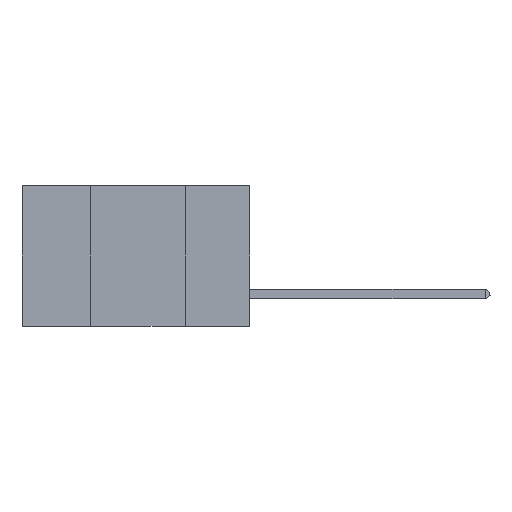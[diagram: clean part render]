
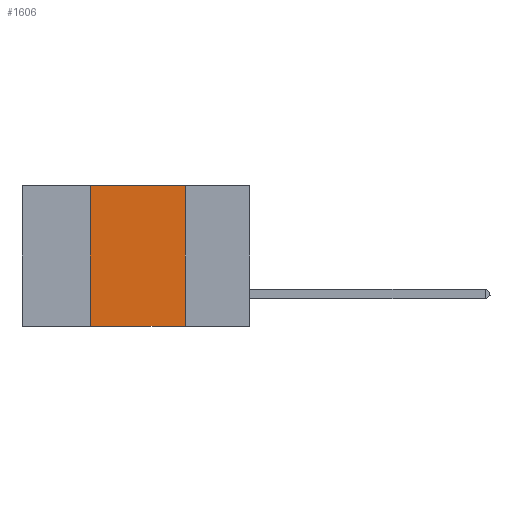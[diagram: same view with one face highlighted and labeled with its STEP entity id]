
A CAD part, left-side view. The second image highlights one B-rep face of the part: STEP entity #1606.
In plain terms, the highlighted planar face has unit normal (-1, 0, 0).
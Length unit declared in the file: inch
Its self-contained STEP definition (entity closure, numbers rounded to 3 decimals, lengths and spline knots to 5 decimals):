
#1122 = DIRECTION ( 'NONE',  ( 0., 0., 1. ) ) ;
#1606 = ADVANCED_FACE ( 'NONE', ( #5337 ), #13560, .F. ) ;
#1828 = VECTOR ( 'NONE', #7093, 39.37008 ) ;
#2267 = VECTOR ( 'NONE', #9466, 39.37008 ) ;
#2295 = DIRECTION ( 'NONE',  ( 0., 0., -1. ) ) ;
#2618 = ORIENTED_EDGE ( 'NONE', *, *, #14950, .F. ) ;
#2641 = VERTEX_POINT ( 'NONE', #3969 ) ;
#2904 = CARTESIAN_POINT ( 'NONE',  ( 0., 0.42, 0. ) ) ;
#3219 = VECTOR ( 'NONE', #8983, 39.37008 ) ;
#3521 = VERTEX_POINT ( 'NONE', #3527 ) ;
#3527 = CARTESIAN_POINT ( 'NONE',  ( 0., 0.17, 0. ) ) ;
#3969 = CARTESIAN_POINT ( 'NONE',  ( 0., 0.42, -0.37 ) ) ;
#5029 = LINE ( 'NONE', #10682, #2267 ) ;
#5337 = FACE_OUTER_BOUND ( 'NONE', #7683, .T. ) ;
#5356 = CARTESIAN_POINT ( 'NONE',  ( 0., 0.17, 0. ) ) ;
#5811 = EDGE_CURVE ( 'NONE', #2641, #11829, #10125, .T. ) ;
#5831 = CARTESIAN_POINT ( 'NONE',  ( 0., 0.6, 0. ) ) ;
#6199 = CARTESIAN_POINT ( 'NONE',  ( 0., 0.6, 0. ) ) ;
#7093 = DIRECTION ( 'NONE',  ( 0., -1., 0. ) ) ;
#7454 = CARTESIAN_POINT ( 'NONE',  ( 0., 0.42, 0. ) ) ;
#7464 = DIRECTION ( 'NONE',  ( 1., 0., 0. ) ) ;
#7683 = EDGE_LOOP ( 'NONE', ( #2618, #15539, #8448, #9654 ) ) ;
#8448 = ORIENTED_EDGE ( 'NONE', *, *, #5811, .F. ) ;
#8983 = DIRECTION ( 'NONE',  ( 0., 0., -1. ) ) ;
#9212 = VERTEX_POINT ( 'NONE', #10717 ) ;
#9373 = VECTOR ( 'NONE', #1122, 39.37008 ) ;
#9466 = DIRECTION ( 'NONE',  ( 0., -1., 0. ) ) ;
#9654 = ORIENTED_EDGE ( 'NONE', *, *, #12715, .T. ) ;
#9865 = LINE ( 'NONE', #5831, #1828 ) ;
#10125 = LINE ( 'NONE', #7454, #9373 ) ;
#10682 = CARTESIAN_POINT ( 'NONE',  ( 0., 0.6, -0.37 ) ) ;
#10717 = CARTESIAN_POINT ( 'NONE',  ( 0., 0.17, -0.37 ) ) ;
#11829 = VERTEX_POINT ( 'NONE', #2904 ) ;
#12715 = EDGE_CURVE ( 'NONE', #2641, #9212, #5029, .T. ) ;
#13560 = PLANE ( 'NONE',  #15586 ) ;
#14950 = EDGE_CURVE ( 'NONE', #3521, #9212, #15178, .T. ) ;
#15178 = LINE ( 'NONE', #5356, #3219 ) ;
#15285 = EDGE_CURVE ( 'NONE', #11829, #3521, #9865, .T. ) ;
#15539 = ORIENTED_EDGE ( 'NONE', *, *, #15285, .F. ) ;
#15586 = AXIS2_PLACEMENT_3D ( 'NONE', #6199, #7464, #2295 ) ;
